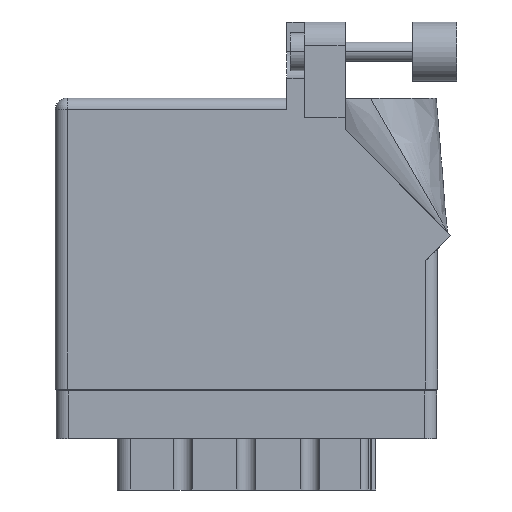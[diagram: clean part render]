
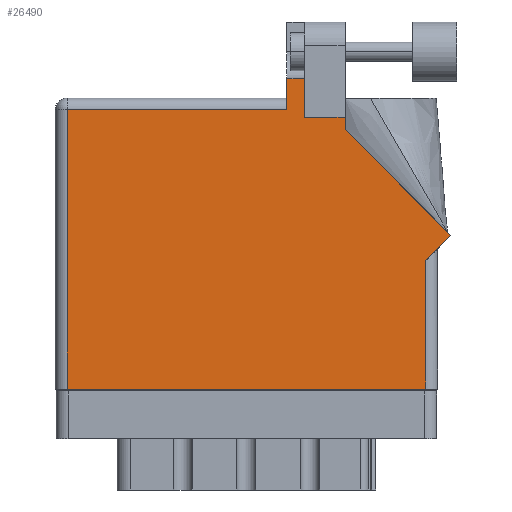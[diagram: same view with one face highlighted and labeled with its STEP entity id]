
A CAD part, front view. The second image highlights one B-rep face of the part: STEP entity #26490.
In plain terms, the highlighted face is planar.
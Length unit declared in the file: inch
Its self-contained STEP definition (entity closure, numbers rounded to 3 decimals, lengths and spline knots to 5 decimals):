
#446 = LINE ( 'NONE', #11308, #2279 ) ;
#795 = CARTESIAN_POINT ( 'NONE',  ( 1.524, 1.43, 0. ) ) ;
#941 = DIRECTION ( 'NONE',  ( 0.707, 0.707, 0. ) ) ;
#1583 = ORIENTED_EDGE ( 'NONE', *, *, #7967, .T. ) ;
#1719 = VERTEX_POINT ( 'NONE', #25817 ) ;
#2279 = VECTOR ( 'NONE', #31836, 39.37008 ) ;
#2614 = VECTOR ( 'NONE', #941, 39.37008 ) ;
#3586 = CARTESIAN_POINT ( 'NONE',  ( 0., 1.468, 0. ) ) ;
#4086 = DIRECTION ( 'NONE',  ( -1., 0., 0. ) ) ;
#4221 = LINE ( 'NONE', #35012, #31863 ) ;
#4363 = VERTEX_POINT ( 'NONE', #28385 ) ;
#4495 = ORIENTED_EDGE ( 'NONE', *, *, #35972, .T. ) ;
#4544 = CARTESIAN_POINT ( 'NONE',  ( 1.948, 0., 0. ) ) ;
#4549 = VECTOR ( 'NONE', #30331, 39.37008 ) ;
#5067 = ORIENTED_EDGE ( 'NONE', *, *, #13544, .T. ) ;
#5479 = CARTESIAN_POINT ( 'NONE',  ( 1.524, 1.36442, 0. ) ) ;
#5611 = DIRECTION ( 'NONE',  ( 0., 1., 0. ) ) ;
#6263 = LINE ( 'NONE', #3586, #28490 ) ;
#6388 = LINE ( 'NONE', #33115, #4549 ) ;
#6409 = VERTEX_POINT ( 'NONE', #10850 ) ;
#6592 = DIRECTION ( 'NONE',  ( 0., 1., 0. ) ) ;
#6720 = CARTESIAN_POINT ( 'NONE',  ( 1.311, 1.43, 0. ) ) ;
#6869 = DIRECTION ( 'NONE',  ( -0.707, 0.707, 0. ) ) ;
#7241 = CARTESIAN_POINT ( 'NONE',  ( 2.08071, 0.80771, 0. ) ) ;
#7610 = ORIENTED_EDGE ( 'NONE', *, *, #24785, .T. ) ;
#7715 = CARTESIAN_POINT ( 'NONE',  ( 1.217, 1.6315, 0. ) ) ;
#7747 = EDGE_CURVE ( 'NONE', #11599, #19877, #6388, .T. ) ;
#7967 = EDGE_CURVE ( 'NONE', #1719, #30553, #32204, .T. ) ;
#8819 = EDGE_CURVE ( 'NONE', #6409, #27386, #18546, .T. ) ;
#9262 = EDGE_CURVE ( 'NONE', #34552, #14679, #34867, .T. ) ;
#9338 = CARTESIAN_POINT ( 'NONE',  ( 2.01, 0.737, 0. ) ) ;
#10570 = VERTEX_POINT ( 'NONE', #26159 ) ;
#10850 = CARTESIAN_POINT ( 'NONE',  ( 1.948, 0.675, 0. ) ) ;
#11168 = CARTESIAN_POINT ( 'NONE',  ( 0.062, 0., 0. ) ) ;
#11207 = ORIENTED_EDGE ( 'NONE', *, *, #25685, .T. ) ;
#11308 = CARTESIAN_POINT ( 'NONE',  ( 1.64177, 1.6315, 0. ) ) ;
#11599 = VERTEX_POINT ( 'NONE', #7715 ) ;
#13544 = EDGE_CURVE ( 'NONE', #27386, #34552, #15131, .T. ) ;
#14083 = VECTOR ( 'NONE', #31194, 39.37008 ) ;
#14460 = VECTOR ( 'NONE', #5611, 39.37008 ) ;
#14679 = VERTEX_POINT ( 'NONE', #795 ) ;
#15131 = LINE ( 'NONE', #7241, #29132 ) ;
#15342 = CARTESIAN_POINT ( 'NONE',  ( 0., 0., 0. ) ) ;
#15546 = VERTEX_POINT ( 'NONE', #4544 ) ;
#15645 = VECTOR ( 'NONE', #6592, 39.37008 ) ;
#15788 = CARTESIAN_POINT ( 'NONE',  ( 1.524, 1.36442, 0. ) ) ;
#16242 = ORIENTED_EDGE ( 'NONE', *, *, #9262, .T. ) ;
#16707 = CARTESIAN_POINT ( 'NONE',  ( 0.062, 0., 0. ) ) ;
#17062 = AXIS2_PLACEMENT_3D ( 'NONE', #36685, #22470, #19804 ) ;
#17637 = ORIENTED_EDGE ( 'NONE', *, *, #7747, .T. ) ;
#18546 = LINE ( 'NONE', #9338, #2614 ) ;
#18935 = PLANE ( 'NONE',  #17062 ) ;
#19804 = DIRECTION ( 'NONE',  ( -1., 0., 0. ) ) ;
#19877 = VERTEX_POINT ( 'NONE', #21738 ) ;
#20776 = DIRECTION ( 'NONE',  ( 0., 1., 0. ) ) ;
#21653 = FACE_OUTER_BOUND ( 'NONE', #26256, .T. ) ;
#21738 = CARTESIAN_POINT ( 'NONE',  ( 1.217, 1.468, 0. ) ) ;
#22470 = DIRECTION ( 'NONE',  ( 0., 0., -1. ) ) ;
#22616 = CARTESIAN_POINT ( 'NONE',  ( 1.524, 1.43, 0. ) ) ;
#23077 = LINE ( 'NONE', #15342, #26704 ) ;
#23656 = ORIENTED_EDGE ( 'NONE', *, *, #37356, .T. ) ;
#24669 = LINE ( 'NONE', #6720, #15645 ) ;
#24785 = EDGE_CURVE ( 'NONE', #10570, #11599, #446, .T. ) ;
#25685 = EDGE_CURVE ( 'NONE', #30553, #15546, #23077, .T. ) ;
#25817 = CARTESIAN_POINT ( 'NONE',  ( 0.062, 1.468, 0. ) ) ;
#26159 = CARTESIAN_POINT ( 'NONE',  ( 1.311, 1.6315, 0. ) ) ;
#26245 = EDGE_CURVE ( 'NONE', #19877, #1719, #6263, .T. ) ;
#26256 = EDGE_LOOP ( 'NONE', ( #37349, #7610, #17637, #31826, #1583, #11207, #4495, #37549, #5067, #16242, #23656 ) ) ;
#26490 = ADVANCED_FACE ( 'NONE', ( #21653 ), #18935, .F. ) ;
#26704 = VECTOR ( 'NONE', #27094, 39.37008 ) ;
#27094 = DIRECTION ( 'NONE',  ( 1., 0., 0. ) ) ;
#27386 = VERTEX_POINT ( 'NONE', #35366 ) ;
#28385 = CARTESIAN_POINT ( 'NONE',  ( 1.311, 1.43, 0. ) ) ;
#28490 = VECTOR ( 'NONE', #4086, 39.37008 ) ;
#28980 = LINE ( 'NONE', #22616, #35807 ) ;
#29132 = VECTOR ( 'NONE', #6869, 39.37008 ) ;
#30331 = DIRECTION ( 'NONE',  ( 0., -1., 0. ) ) ;
#30553 = VERTEX_POINT ( 'NONE', #16707 ) ;
#31096 = DIRECTION ( 'NONE',  ( -1., 0., 0. ) ) ;
#31194 = DIRECTION ( 'NONE',  ( 0., -1., 0. ) ) ;
#31826 = ORIENTED_EDGE ( 'NONE', *, *, #26245, .T. ) ;
#31836 = DIRECTION ( 'NONE',  ( -1., 0., 0. ) ) ;
#31863 = VECTOR ( 'NONE', #20776, 39.37008 ) ;
#32204 = LINE ( 'NONE', #11168, #14083 ) ;
#33115 = CARTESIAN_POINT ( 'NONE',  ( 1.217, 1.53, 0. ) ) ;
#34552 = VERTEX_POINT ( 'NONE', #15788 ) ;
#34867 = LINE ( 'NONE', #5479, #14460 ) ;
#35012 = CARTESIAN_POINT ( 'NONE',  ( 1.948, 0.737, 0. ) ) ;
#35048 = EDGE_CURVE ( 'NONE', #4363, #10570, #24669, .T. ) ;
#35366 = CARTESIAN_POINT ( 'NONE',  ( 2.08071, 0.80771, 0. ) ) ;
#35807 = VECTOR ( 'NONE', #31096, 39.37008 ) ;
#35972 = EDGE_CURVE ( 'NONE', #15546, #6409, #4221, .T. ) ;
#36685 = CARTESIAN_POINT ( 'NONE',  ( 0., 1.53, 0. ) ) ;
#37349 = ORIENTED_EDGE ( 'NONE', *, *, #35048, .T. ) ;
#37356 = EDGE_CURVE ( 'NONE', #14679, #4363, #28980, .T. ) ;
#37549 = ORIENTED_EDGE ( 'NONE', *, *, #8819, .T. ) ;
